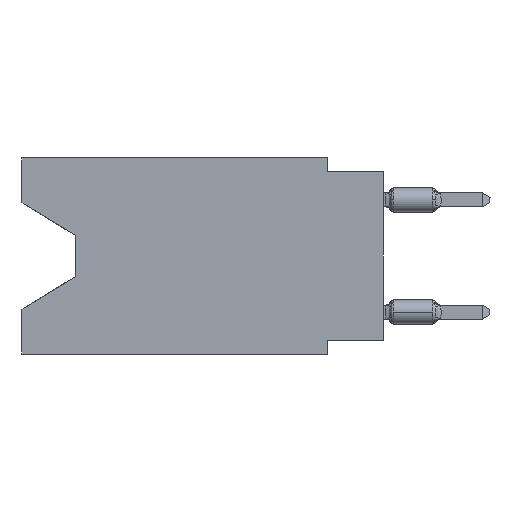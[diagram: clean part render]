
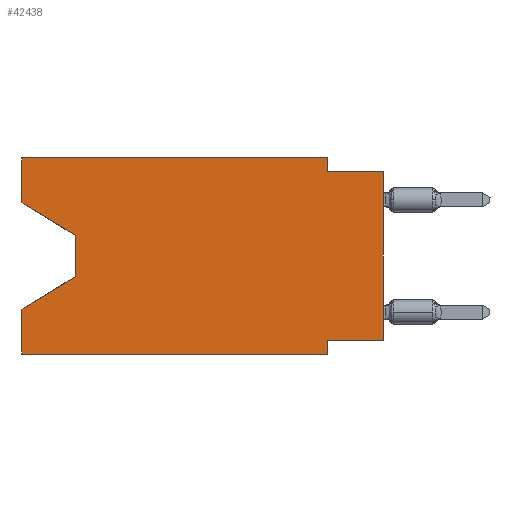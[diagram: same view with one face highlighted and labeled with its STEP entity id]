
A CAD part, left-side view. The second image highlights one B-rep face of the part: STEP entity #42438.
In plain terms, the highlighted planar face has unit normal (-1, 0, 0).
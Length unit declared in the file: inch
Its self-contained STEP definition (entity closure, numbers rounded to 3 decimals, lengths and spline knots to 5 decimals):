
#659 = CARTESIAN_POINT ( 'NONE',  ( 0., 0.645, -0.08025 ) ) ;
#671 = EDGE_CURVE ( 'NONE', #36746, #22360, #34477, .T. ) ;
#1614 = CARTESIAN_POINT ( 'NONE',  ( 0., 0.645, 0. ) ) ;
#2085 = EDGE_LOOP ( 'NONE', ( #38957, #46690, #22447, #26359, #12112, #2713, #15109, #29749, #45952, #14115, #19226, #32941 ) ) ;
#2713 = ORIENTED_EDGE ( 'NONE', *, *, #11877, .F. ) ;
#3653 = VECTOR ( 'NONE', #30839, 39.37008 ) ;
#3939 = DIRECTION ( 'NONE',  ( 0., -0.855, -0.519 ) ) ;
#4565 = LINE ( 'NONE', #44460, #36139 ) ;
#4911 = VECTOR ( 'NONE', #3939, 39.37008 ) ;
#5200 = DIRECTION ( 'NONE',  ( 0., 0., -1. ) ) ;
#5353 = CARTESIAN_POINT ( 'NONE',  ( 0., 0., 0. ) ) ;
#5469 = EDGE_CURVE ( 'NONE', #28006, #8907, #14901, .T. ) ;
#5828 = DIRECTION ( 'NONE',  ( 0., 0.855, -0.519 ) ) ;
#6352 = CARTESIAN_POINT ( 'NONE',  ( 0., 0.1, -0.35 ) ) ;
#6865 = CARTESIAN_POINT ( 'NONE',  ( 0., 0., -0.325 ) ) ;
#8311 = CARTESIAN_POINT ( 'NONE',  ( 0., 0.645, -0.35 ) ) ;
#8907 = VERTEX_POINT ( 'NONE', #12413 ) ;
#9022 = LINE ( 'NONE', #5353, #17078 ) ;
#10041 = DIRECTION ( 'NONE',  ( 0., 0., 1. ) ) ;
#10625 = CARTESIAN_POINT ( 'NONE',  ( 0., 0.1, -0.025 ) ) ;
#11076 = CARTESIAN_POINT ( 'NONE',  ( 0., 0.1, 0. ) ) ;
#11601 = EDGE_CURVE ( 'NONE', #46626, #28000, #4565, .T. ) ;
#11877 = EDGE_CURVE ( 'NONE', #31559, #12788, #27463, .T. ) ;
#12112 = ORIENTED_EDGE ( 'NONE', *, *, #46479, .T. ) ;
#12413 = CARTESIAN_POINT ( 'NONE',  ( 0., 0.55, -0.138 ) ) ;
#12788 = VERTEX_POINT ( 'NONE', #6352 ) ;
#13185 = DIRECTION ( 'NONE',  ( 0., -1., 0. ) ) ;
#13545 = PLANE ( 'NONE',  #21290 ) ;
#13595 = DIRECTION ( 'NONE',  ( 0., 0., 1. ) ) ;
#13930 = CARTESIAN_POINT ( 'NONE',  ( 0., 0.55, -0.212 ) ) ;
#14042 = VERTEX_POINT ( 'NONE', #21818 ) ;
#14115 = ORIENTED_EDGE ( 'NONE', *, *, #30002, .F. ) ;
#14668 = LINE ( 'NONE', #18832, #33677 ) ;
#14803 = LINE ( 'NONE', #26301, #19534 ) ;
#14901 = LINE ( 'NONE', #39378, #4911 ) ;
#15109 = ORIENTED_EDGE ( 'NONE', *, *, #22015, .F. ) ;
#16912 = VECTOR ( 'NONE', #28386, 39.37008 ) ;
#17078 = VECTOR ( 'NONE', #10041, 39.37008 ) ;
#17646 = DIRECTION ( 'NONE',  ( 0., 0., -1. ) ) ;
#17988 = DIRECTION ( 'NONE',  ( 1., 0., 0. ) ) ;
#18174 = CARTESIAN_POINT ( 'NONE',  ( 0., 0.1, 0. ) ) ;
#18832 = CARTESIAN_POINT ( 'NONE',  ( 0., 0.645, 0. ) ) ;
#19226 = ORIENTED_EDGE ( 'NONE', *, *, #38424, .F. ) ;
#19436 = VECTOR ( 'NONE', #31316, 39.37008 ) ;
#19534 = VECTOR ( 'NONE', #30691, 39.37008 ) ;
#19585 = CARTESIAN_POINT ( 'NONE',  ( 0., 0.645, 0. ) ) ;
#19634 = CARTESIAN_POINT ( 'NONE',  ( 0., 0.1, -0.35 ) ) ;
#21290 = AXIS2_PLACEMENT_3D ( 'NONE', #41457, #17988, #5200 ) ;
#21310 = DIRECTION ( 'NONE',  ( 0., 1., 0. ) ) ;
#21818 = CARTESIAN_POINT ( 'NONE',  ( 0., 0.645, -0.35 ) ) ;
#22015 = EDGE_CURVE ( 'NONE', #22673, #31559, #25209, .T. ) ;
#22360 = VERTEX_POINT ( 'NONE', #44713 ) ;
#22447 = ORIENTED_EDGE ( 'NONE', *, *, #671, .T. ) ;
#22673 = VERTEX_POINT ( 'NONE', #6865 ) ;
#25209 = LINE ( 'NONE', #41108, #40772 ) ;
#25217 = VECTOR ( 'NONE', #17646, 39.37008 ) ;
#26301 = CARTESIAN_POINT ( 'NONE',  ( 0., 0.55, -0.138 ) ) ;
#26359 = ORIENTED_EDGE ( 'NONE', *, *, #40705, .F. ) ;
#27077 = VECTOR ( 'NONE', #13595, 39.37008 ) ;
#27421 = LINE ( 'NONE', #19585, #19436 ) ;
#27463 = LINE ( 'NONE', #19634, #3653 ) ;
#27830 = VERTEX_POINT ( 'NONE', #11076 ) ;
#28000 = VERTEX_POINT ( 'NONE', #35849 ) ;
#28006 = VERTEX_POINT ( 'NONE', #659 ) ;
#28386 = DIRECTION ( 'NONE',  ( 0., -1., 0. ) ) ;
#29749 = ORIENTED_EDGE ( 'NONE', *, *, #40044, .T. ) ;
#30002 = EDGE_CURVE ( 'NONE', #27830, #46626, #45037, .T. ) ;
#30691 = DIRECTION ( 'NONE',  ( 0., 0., -1. ) ) ;
#30839 = DIRECTION ( 'NONE',  ( 0., 0., -1. ) ) ;
#31316 = DIRECTION ( 'NONE',  ( 0., -1., 0. ) ) ;
#31559 = VERTEX_POINT ( 'NONE', #33672 ) ;
#32941 = ORIENTED_EDGE ( 'NONE', *, *, #48810, .F. ) ;
#33353 = FACE_OUTER_BOUND ( 'NONE', #2085, .T. ) ;
#33672 = CARTESIAN_POINT ( 'NONE',  ( 0., 0.1, -0.325 ) ) ;
#33677 = VECTOR ( 'NONE', #42314, 39.37008 ) ;
#34477 = LINE ( 'NONE', #13930, #35119 ) ;
#35119 = VECTOR ( 'NONE', #5828, 39.37008 ) ;
#35849 = CARTESIAN_POINT ( 'NONE',  ( 0., 0., -0.025 ) ) ;
#36139 = VECTOR ( 'NONE', #13185, 39.37008 ) ;
#36746 = VERTEX_POINT ( 'NONE', #43366 ) ;
#38424 = EDGE_CURVE ( 'NONE', #46604, #27830, #27421, .T. ) ;
#38957 = ORIENTED_EDGE ( 'NONE', *, *, #5469, .T. ) ;
#39378 = CARTESIAN_POINT ( 'NONE',  ( 0., 0.645, -0.08025 ) ) ;
#40044 = EDGE_CURVE ( 'NONE', #22673, #28000, #9022, .T. ) ;
#40705 = EDGE_CURVE ( 'NONE', #14042, #22360, #45149, .T. ) ;
#40772 = VECTOR ( 'NONE', #21310, 39.37008 ) ;
#41108 = CARTESIAN_POINT ( 'NONE',  ( 0., 0., -0.325 ) ) ;
#41457 = CARTESIAN_POINT ( 'NONE',  ( 0., 0.645, 0. ) ) ;
#42314 = DIRECTION ( 'NONE',  ( 0., 0., 1. ) ) ;
#42438 = ADVANCED_FACE ( 'NONE', ( #33353 ), #13545, .F. ) ;
#43366 = CARTESIAN_POINT ( 'NONE',  ( 0., 0.55, -0.212 ) ) ;
#44031 = LINE ( 'NONE', #8311, #16912 ) ;
#44460 = CARTESIAN_POINT ( 'NONE',  ( 0., 0., -0.025 ) ) ;
#44713 = CARTESIAN_POINT ( 'NONE',  ( 0., 0.645, -0.26975 ) ) ;
#45037 = LINE ( 'NONE', #18174, #25217 ) ;
#45149 = LINE ( 'NONE', #1614, #27077 ) ;
#45829 = CARTESIAN_POINT ( 'NONE',  ( 0., 0.645, 0. ) ) ;
#45952 = ORIENTED_EDGE ( 'NONE', *, *, #11601, .F. ) ;
#46479 = EDGE_CURVE ( 'NONE', #14042, #12788, #44031, .T. ) ;
#46604 = VERTEX_POINT ( 'NONE', #45829 ) ;
#46626 = VERTEX_POINT ( 'NONE', #10625 ) ;
#46690 = ORIENTED_EDGE ( 'NONE', *, *, #49062, .T. ) ;
#48810 = EDGE_CURVE ( 'NONE', #28006, #46604, #14668, .T. ) ;
#49062 = EDGE_CURVE ( 'NONE', #8907, #36746, #14803, .T. ) ;
